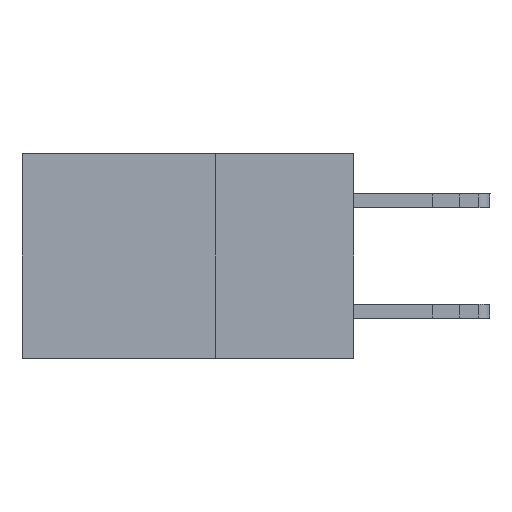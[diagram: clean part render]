
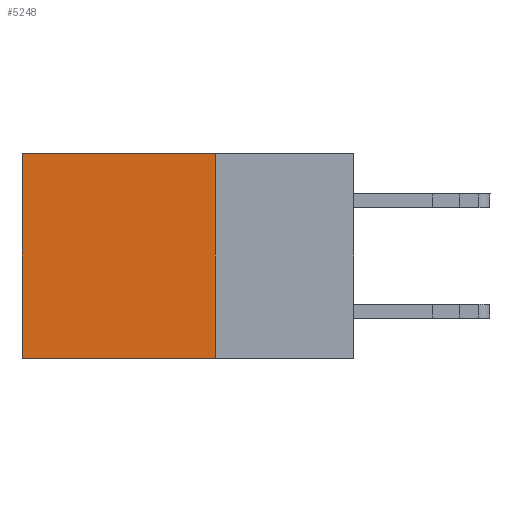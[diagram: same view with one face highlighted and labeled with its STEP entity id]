
A CAD part, left-side view. The second image highlights one B-rep face of the part: STEP entity #5248.
In plain terms, the highlighted planar face has unit normal (-1, 0, 0).
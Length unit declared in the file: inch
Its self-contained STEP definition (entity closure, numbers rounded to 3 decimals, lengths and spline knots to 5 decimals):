
#1144 = EDGE_CURVE ( 'NONE', #16063, #10018, #14911, .T. ) ;
#1628 = CARTESIAN_POINT ( 'NONE',  ( 0.2875, 0.6, 0. ) ) ;
#1803 = CARTESIAN_POINT ( 'NONE',  ( 0.2875, 0.25, 0. ) ) ;
#4427 = CARTESIAN_POINT ( 'NONE',  ( 0.2875, 0.25, -0.37 ) ) ;
#4735 = ORIENTED_EDGE ( 'NONE', *, *, #17880, .T. ) ;
#5120 = CARTESIAN_POINT ( 'NONE',  ( 0.2875, 0.6, -0.37 ) ) ;
#5193 = CARTESIAN_POINT ( 'NONE',  ( 0.2875, 0.25, 0. ) ) ;
#5246 = EDGE_LOOP ( 'NONE', ( #12236, #13236, #6957, #4735 ) ) ;
#5248 = ADVANCED_FACE ( 'NONE', ( #15513 ), #6878, .F. ) ;
#6099 = VECTOR ( 'NONE', #19966, 39.37008 ) ;
#6878 = PLANE ( 'NONE',  #17915 ) ;
#6957 = ORIENTED_EDGE ( 'NONE', *, *, #20288, .F. ) ;
#7074 = CARTESIAN_POINT ( 'NONE',  ( 0.2875, 0.25, 0. ) ) ;
#7550 = VECTOR ( 'NONE', #12794, 39.37008 ) ;
#8519 = DIRECTION ( 'NONE',  ( 1., 0., 0. ) ) ;
#9254 = LINE ( 'NONE', #1803, #16860 ) ;
#10018 = VERTEX_POINT ( 'NONE', #5120 ) ;
#11178 = CARTESIAN_POINT ( 'NONE',  ( 0.2875, 0.25, -0.37 ) ) ;
#12191 = CARTESIAN_POINT ( 'NONE',  ( 0.2875, 0.25, 0. ) ) ;
#12236 = ORIENTED_EDGE ( 'NONE', *, *, #1144, .T. ) ;
#12794 = DIRECTION ( 'NONE',  ( 0., 1., 0. ) ) ;
#12869 = VERTEX_POINT ( 'NONE', #4427 ) ;
#13236 = ORIENTED_EDGE ( 'NONE', *, *, #15216, .F. ) ;
#13328 = VERTEX_POINT ( 'NONE', #12191 ) ;
#13347 = DIRECTION ( 'NONE',  ( 0., 0., -1. ) ) ;
#14279 = LINE ( 'NONE', #7074, #6099 ) ;
#14911 = LINE ( 'NONE', #20126, #19104 ) ;
#15216 = EDGE_CURVE ( 'NONE', #12869, #10018, #20391, .T. ) ;
#15513 = FACE_OUTER_BOUND ( 'NONE', #5246, .T. ) ;
#16063 = VERTEX_POINT ( 'NONE', #1628 ) ;
#16860 = VECTOR ( 'NONE', #13347, 39.37008 ) ;
#17880 = EDGE_CURVE ( 'NONE', #13328, #16063, #14279, .T. ) ;
#17915 = AXIS2_PLACEMENT_3D ( 'NONE', #5193, #8519, #19781 ) ;
#19104 = VECTOR ( 'NONE', #20693, 39.37008 ) ;
#19781 = DIRECTION ( 'NONE',  ( 0., 0., -1. ) ) ;
#19966 = DIRECTION ( 'NONE',  ( 0., 1., 0. ) ) ;
#20126 = CARTESIAN_POINT ( 'NONE',  ( 0.2875, 0.6, 0. ) ) ;
#20288 = EDGE_CURVE ( 'NONE', #13328, #12869, #9254, .T. ) ;
#20391 = LINE ( 'NONE', #11178, #7550 ) ;
#20693 = DIRECTION ( 'NONE',  ( 0., 0., -1. ) ) ;
